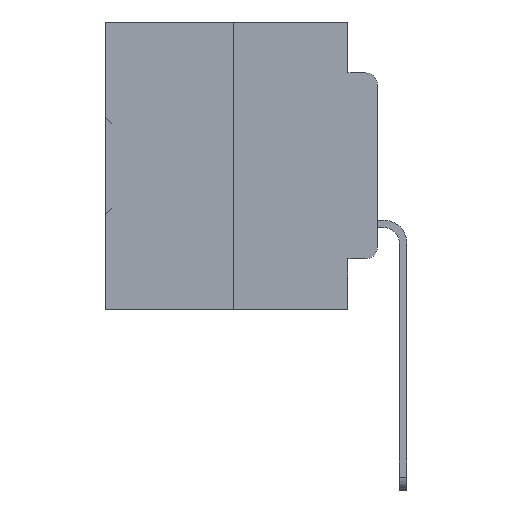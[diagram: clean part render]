
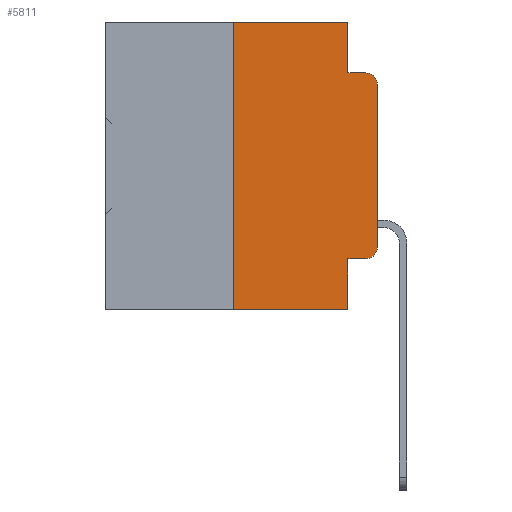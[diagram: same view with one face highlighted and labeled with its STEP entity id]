
A CAD part, left-side view. The second image highlights one B-rep face of the part: STEP entity #5811.
In plain terms, the highlighted planar face has unit normal (-1, 0, 0).
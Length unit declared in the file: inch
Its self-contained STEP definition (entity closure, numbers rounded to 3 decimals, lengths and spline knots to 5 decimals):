
#1278 = CARTESIAN_POINT ( 'NONE',  ( 0., 0., -0.1085 ) ) ;
#1491 = ORIENTED_EDGE ( 'NONE', *, *, #21002, .F. ) ;
#2018 = ORIENTED_EDGE ( 'NONE', *, *, #16922, .T. ) ;
#2065 = CARTESIAN_POINT ( 'NONE',  ( 0., 0.051, -0.0885 ) ) ;
#3288 = VECTOR ( 'NONE', #7816, 39.37008 ) ;
#4371 = VERTEX_POINT ( 'NONE', #39290 ) ;
#4454 = CARTESIAN_POINT ( 'NONE',  ( 0., 0.02, -0.3915 ) ) ;
#4482 = PLANE ( 'NONE',  #19227 ) ;
#4505 = ORIENTED_EDGE ( 'NONE', *, *, #23018, .F. ) ;
#5089 = DIRECTION ( 'NONE',  ( 0., 0., -1. ) ) ;
#5195 = LINE ( 'NONE', #37663, #13380 ) ;
#5209 = LINE ( 'NONE', #16453, #36421 ) ;
#5811 = ADVANCED_FACE ( 'NONE', ( #13400 ), #4482, .F. ) ;
#5876 = EDGE_CURVE ( 'NONE', #4371, #23529, #19568, .T. ) ;
#6087 = VECTOR ( 'NONE', #26788, 39.37008 ) ;
#6355 = DIRECTION ( 'NONE',  ( 0., -1., 0. ) ) ;
#7512 = DIRECTION ( 'NONE',  ( 0., 0., -1. ) ) ;
#7544 = DIRECTION ( 'NONE',  ( 1., 0., 0. ) ) ;
#7755 = VERTEX_POINT ( 'NONE', #37419 ) ;
#7816 = DIRECTION ( 'NONE',  ( 0., 0., 1. ) ) ;
#9415 = DIRECTION ( 'NONE',  ( 0., -1., 0. ) ) ;
#10673 = VECTOR ( 'NONE', #5089, 39.37008 ) ;
#10796 = EDGE_CURVE ( 'NONE', #38686, #4371, #19073, .T. ) ;
#11233 = ORIENTED_EDGE ( 'NONE', *, *, #29041, .F. ) ;
#11725 = AXIS2_PLACEMENT_3D ( 'NONE', #4454, #25749, #7512 ) ;
#11876 = EDGE_CURVE ( 'NONE', #15020, #21654, #35388, .T. ) ;
#13179 = VERTEX_POINT ( 'NONE', #14141 ) ;
#13380 = VECTOR ( 'NONE', #25640, 39.37008 ) ;
#13400 = FACE_OUTER_BOUND ( 'NONE', #21446, .T. ) ;
#13925 = VERTEX_POINT ( 'NONE', #29617 ) ;
#13967 = LINE ( 'NONE', #2065, #14899 ) ;
#14113 = VERTEX_POINT ( 'NONE', #18694 ) ;
#14141 = CARTESIAN_POINT ( 'NONE',  ( 0., 0.051, -0.0885 ) ) ;
#14899 = VECTOR ( 'NONE', #38240, 39.37008 ) ;
#15020 = VERTEX_POINT ( 'NONE', #25880 ) ;
#15661 = DIRECTION ( 'NONE',  ( -1., 0., 0. ) ) ;
#16453 = CARTESIAN_POINT ( 'NONE',  ( 0., 0.051, 0. ) ) ;
#16909 = ORIENTED_EDGE ( 'NONE', *, *, #5876, .T. ) ;
#16922 = EDGE_CURVE ( 'NONE', #7755, #38686, #19500, .T. ) ;
#17548 = CIRCLE ( 'NONE', #22731, 0.02 ) ;
#18694 = CARTESIAN_POINT ( 'NONE',  ( 0., 0.02, -0.0885 ) ) ;
#19073 = CIRCLE ( 'NONE', #11725, 0.02 ) ;
#19227 = AXIS2_PLACEMENT_3D ( 'NONE', #25779, #7544, #28789 ) ;
#19449 = VECTOR ( 'NONE', #6355, 39.37008 ) ;
#19500 = LINE ( 'NONE', #20736, #6087 ) ;
#19568 = LINE ( 'NONE', #37929, #3288 ) ;
#20319 = CARTESIAN_POINT ( 'NONE',  ( 0., 0.051, 0. ) ) ;
#20736 = CARTESIAN_POINT ( 'NONE',  ( 0., 0.051, -0.4115 ) ) ;
#21002 = EDGE_CURVE ( 'NONE', #7755, #21654, #28655, .T. ) ;
#21327 = LINE ( 'NONE', #36438, #39091 ) ;
#21446 = EDGE_LOOP ( 'NONE', ( #16909, #32890, #35714, #11233, #24040, #4505, #30597, #1491, #2018, #26385 ) ) ;
#21654 = VERTEX_POINT ( 'NONE', #28104 ) ;
#22731 = AXIS2_PLACEMENT_3D ( 'NONE', #33630, #15661, #36640 ) ;
#23018 = EDGE_CURVE ( 'NONE', #15020, #38838, #5195, .T. ) ;
#23529 = VERTEX_POINT ( 'NONE', #1278 ) ;
#24040 = ORIENTED_EDGE ( 'NONE', *, *, #24334, .F. ) ;
#24334 = EDGE_CURVE ( 'NONE', #38838, #13925, #21327, .T. ) ;
#24361 = CARTESIAN_POINT ( 'NONE',  ( 0., 0.02, -0.4115 ) ) ;
#25640 = DIRECTION ( 'NONE',  ( 0., 0., 1. ) ) ;
#25749 = DIRECTION ( 'NONE',  ( -1., 0., 0. ) ) ;
#25779 = CARTESIAN_POINT ( 'NONE',  ( 0., 0.473, 0. ) ) ;
#25880 = CARTESIAN_POINT ( 'NONE',  ( 0., 0.25, -0.5 ) ) ;
#26385 = ORIENTED_EDGE ( 'NONE', *, *, #10796, .T. ) ;
#26788 = DIRECTION ( 'NONE',  ( 0., -1., 0. ) ) ;
#28104 = CARTESIAN_POINT ( 'NONE',  ( 0., 0.051, -0.5 ) ) ;
#28655 = LINE ( 'NONE', #20319, #10673 ) ;
#28789 = DIRECTION ( 'NONE',  ( 0., 0., -1. ) ) ;
#29041 = EDGE_CURVE ( 'NONE', #13925, #13179, #5209, .T. ) ;
#29617 = CARTESIAN_POINT ( 'NONE',  ( 0., 0.051, 0. ) ) ;
#30489 = CARTESIAN_POINT ( 'NONE',  ( 0., 0.473, -0.5 ) ) ;
#30597 = ORIENTED_EDGE ( 'NONE', *, *, #11876, .T. ) ;
#32890 = ORIENTED_EDGE ( 'NONE', *, *, #35049, .T. ) ;
#33027 = EDGE_CURVE ( 'NONE', #13179, #14113, #13967, .T. ) ;
#33630 = CARTESIAN_POINT ( 'NONE',  ( 0., 0.02, -0.1085 ) ) ;
#34003 = CARTESIAN_POINT ( 'NONE',  ( 0., 0.25, 0. ) ) ;
#34446 = DIRECTION ( 'NONE',  ( 0., 0., -1. ) ) ;
#35049 = EDGE_CURVE ( 'NONE', #23529, #14113, #17548, .T. ) ;
#35388 = LINE ( 'NONE', #30489, #19449 ) ;
#35714 = ORIENTED_EDGE ( 'NONE', *, *, #33027, .F. ) ;
#36421 = VECTOR ( 'NONE', #34446, 39.37008 ) ;
#36438 = CARTESIAN_POINT ( 'NONE',  ( 0., 0.473, 0. ) ) ;
#36640 = DIRECTION ( 'NONE',  ( 0., 0., -1. ) ) ;
#37419 = CARTESIAN_POINT ( 'NONE',  ( 0., 0.051, -0.4115 ) ) ;
#37663 = CARTESIAN_POINT ( 'NONE',  ( 0., 0.25, 0. ) ) ;
#37929 = CARTESIAN_POINT ( 'NONE',  ( 0., 0., 0. ) ) ;
#38240 = DIRECTION ( 'NONE',  ( 0., -1., 0. ) ) ;
#38686 = VERTEX_POINT ( 'NONE', #24361 ) ;
#38838 = VERTEX_POINT ( 'NONE', #34003 ) ;
#39091 = VECTOR ( 'NONE', #9415, 39.37008 ) ;
#39290 = CARTESIAN_POINT ( 'NONE',  ( 0., 0., -0.3915 ) ) ;
